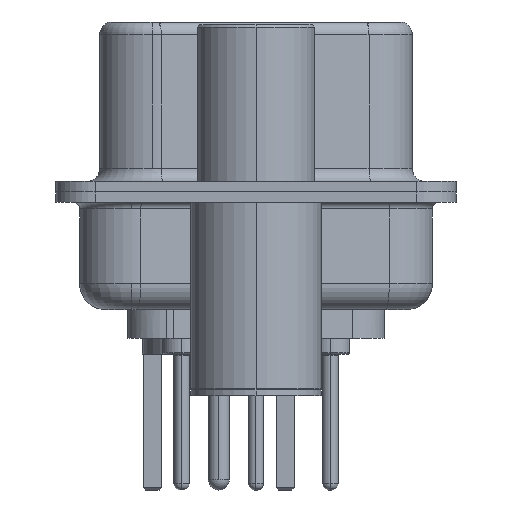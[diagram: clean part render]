
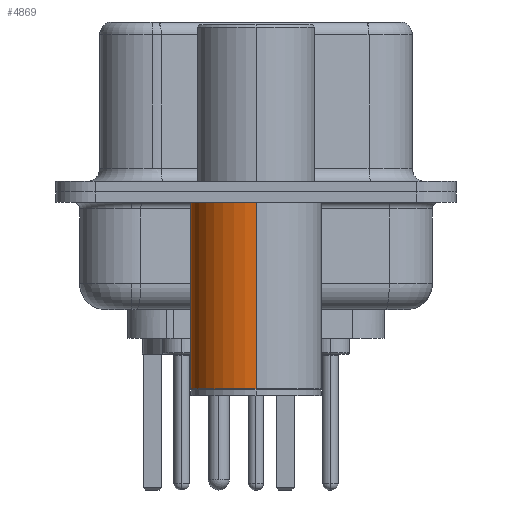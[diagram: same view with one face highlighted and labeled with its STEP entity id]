
A CAD part, left-side view. The second image highlights one B-rep face of the part: STEP entity #4869.
In plain terms, the highlighted cylindrical face has radius 2.5 mm (diameter 5 mm), a partial arc.
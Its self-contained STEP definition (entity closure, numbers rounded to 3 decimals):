
#1077 = VERTEX_POINT ( 'NONE', #21153 ) ;
#1585 = ORIENTED_EDGE ( 'NONE', *, *, #27561, .F. ) ;
#1603 = FACE_OUTER_BOUND ( 'NONE', #33801, .T. ) ;
#4852 = AXIS2_PLACEMENT_3D ( 'NONE', #5379, #26525, #8433 ) ;
#4869 = ADVANCED_FACE ( 'NONE', ( #1603 ), #16723, .T. ) ;
#5156 = CARTESIAN_POINT ( 'NONE',  ( -2.5, 0., -7.525 ) ) ;
#5379 = CARTESIAN_POINT ( 'NONE',  ( 0., 0., -0.4 ) ) ;
#5804 = VERTEX_POINT ( 'NONE', #24883 ) ;
#7360 = EDGE_CURVE ( 'NONE', #1077, #5804, #22310, .T. ) ;
#8294 = VERTEX_POINT ( 'NONE', #5156 ) ;
#8433 = DIRECTION ( 'NONE',  ( 1., 0., 0. ) ) ;
#9273 = ORIENTED_EDGE ( 'NONE', *, *, #12738, .T. ) ;
#10415 = DIRECTION ( 'NONE',  ( 0., 0., 1. ) ) ;
#12442 = DIRECTION ( 'NONE',  ( 0., 0., 1. ) ) ;
#12738 = EDGE_CURVE ( 'NONE', #1077, #8294, #15813, .T. ) ;
#13055 = CARTESIAN_POINT ( 'NONE',  ( 2.5, 0., 0.581 ) ) ;
#13091 = CARTESIAN_POINT ( 'NONE',  ( 0., 0., 0.581 ) ) ;
#15197 = VECTOR ( 'NONE', #31140, 1000. ) ;
#15518 = CIRCLE ( 'NONE', #4852, 2.5 ) ;
#15813 = CIRCLE ( 'NONE', #38170, 2.5 ) ;
#16570 = DIRECTION ( 'NONE',  ( 0., 0., 1. ) ) ;
#16723 = CYLINDRICAL_SURFACE ( 'NONE', #21311, 2.5 ) ;
#18117 = EDGE_CURVE ( 'NONE', #8294, #19055, #35836, .T. ) ;
#18522 = CARTESIAN_POINT ( 'NONE',  ( -2.5, 0., 0.581 ) ) ;
#19055 = VERTEX_POINT ( 'NONE', #19837 ) ;
#19837 = CARTESIAN_POINT ( 'NONE',  ( -2.5, 0., -0.4 ) ) ;
#21153 = CARTESIAN_POINT ( 'NONE',  ( 2.5, 0., -7.525 ) ) ;
#21311 = AXIS2_PLACEMENT_3D ( 'NONE', #13091, #10415, #35516 ) ;
#22310 = LINE ( 'NONE', #13055, #15197 ) ;
#24883 = CARTESIAN_POINT ( 'NONE',  ( 2.5, 0., -0.4 ) ) ;
#25414 = ORIENTED_EDGE ( 'NONE', *, *, #7360, .F. ) ;
#25900 = VECTOR ( 'NONE', #12442, 1000. ) ;
#26525 = DIRECTION ( 'NONE',  ( 0., 0., 1. ) ) ;
#27561 = EDGE_CURVE ( 'NONE', #5804, #19055, #15518, .T. ) ;
#28249 = ORIENTED_EDGE ( 'NONE', *, *, #18117, .T. ) ;
#31140 = DIRECTION ( 'NONE',  ( 0., 0., 1. ) ) ;
#33801 = EDGE_LOOP ( 'NONE', ( #9273, #28249, #1585, #25414 ) ) ;
#34643 = CARTESIAN_POINT ( 'NONE',  ( 0., 0., -7.525 ) ) ;
#35516 = DIRECTION ( 'NONE',  ( 1., 0., 0. ) ) ;
#35836 = LINE ( 'NONE', #18522, #25900 ) ;
#37702 = DIRECTION ( 'NONE',  ( 1., 0., 0. ) ) ;
#38170 = AXIS2_PLACEMENT_3D ( 'NONE', #34643, #16570, #37702 ) ;
